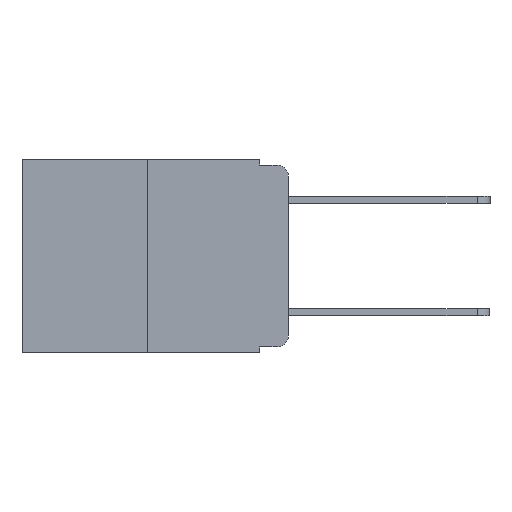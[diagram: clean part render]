
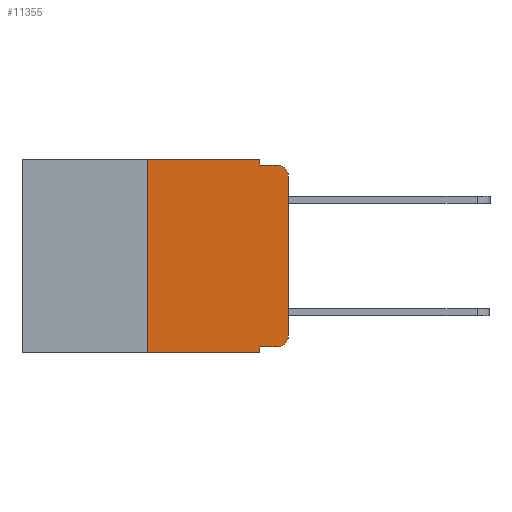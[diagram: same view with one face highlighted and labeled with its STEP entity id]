
A CAD part, left-side view. The second image highlights one B-rep face of the part: STEP entity #11355.
In plain terms, the highlighted planar face has unit normal (-1, 0, 0).
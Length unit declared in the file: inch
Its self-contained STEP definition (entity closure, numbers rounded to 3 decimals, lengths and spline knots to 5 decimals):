
#37 = ORIENTED_EDGE ( 'NONE', *, *, #12693, .T. ) ;
#157 = CARTESIAN_POINT ( 'NONE',  ( 0., 0.25, 0. ) ) ;
#374 = CARTESIAN_POINT ( 'NONE',  ( 0., 0.051, -0.01 ) ) ;
#707 = DIRECTION ( 'NONE',  ( 0., 0., -1. ) ) ;
#834 = CARTESIAN_POINT ( 'NONE',  ( 0., 0.02, -0.01 ) ) ;
#868 = EDGE_CURVE ( 'NONE', #13894, #13662, #4724, .T. ) ;
#949 = FACE_OUTER_BOUND ( 'NONE', #23629, .T. ) ;
#1075 = ORIENTED_EDGE ( 'NONE', *, *, #868, .F. ) ;
#1116 = VERTEX_POINT ( 'NONE', #12296 ) ;
#2257 = ORIENTED_EDGE ( 'NONE', *, *, #14462, .F. ) ;
#2414 = DIRECTION ( 'NONE',  ( 0., -1., 0. ) ) ;
#3928 = VERTEX_POINT ( 'NONE', #18220 ) ;
#4373 = LINE ( 'NONE', #13932, #23653 ) ;
#4468 = VECTOR ( 'NONE', #23866, 39.37008 ) ;
#4724 = LINE ( 'NONE', #21136, #17749 ) ;
#4776 = DIRECTION ( 'NONE',  ( -1., 0., 0. ) ) ;
#5752 = ORIENTED_EDGE ( 'NONE', *, *, #17588, .F. ) ;
#6073 = CIRCLE ( 'NONE', #23241, 0.02 ) ;
#6111 = VERTEX_POINT ( 'NONE', #834 ) ;
#6170 = ORIENTED_EDGE ( 'NONE', *, *, #16269, .T. ) ;
#6327 = DIRECTION ( 'NONE',  ( 1., 0., 0. ) ) ;
#6412 = CARTESIAN_POINT ( 'NONE',  ( 0., 0.473, 0. ) ) ;
#6756 = EDGE_CURVE ( 'NONE', #9820, #3928, #8186, .T. ) ;
#6792 = DIRECTION ( 'NONE',  ( 0., 0., 1. ) ) ;
#7317 = VERTEX_POINT ( 'NONE', #8262 ) ;
#7321 = VECTOR ( 'NONE', #14091, 39.37008 ) ;
#7469 = CIRCLE ( 'NONE', #14617, 0.02 ) ;
#7599 = VECTOR ( 'NONE', #707, 39.37008 ) ;
#7732 = DIRECTION ( 'NONE',  ( 0., 0., -1. ) ) ;
#8186 = LINE ( 'NONE', #16367, #7599 ) ;
#8262 = CARTESIAN_POINT ( 'NONE',  ( 0., 0.25, -0.343 ) ) ;
#8353 = PLANE ( 'NONE',  #20276 ) ;
#8526 = CARTESIAN_POINT ( 'NONE',  ( 0., 0.02, -0.03 ) ) ;
#8657 = EDGE_CURVE ( 'NONE', #7317, #3928, #4373, .T. ) ;
#8897 = ORIENTED_EDGE ( 'NONE', *, *, #8657, .T. ) ;
#9194 = DIRECTION ( 'NONE',  ( 0., -1., 0. ) ) ;
#9333 = EDGE_CURVE ( 'NONE', #7317, #13700, #9675, .T. ) ;
#9458 = VECTOR ( 'NONE', #2414, 39.37008 ) ;
#9675 = LINE ( 'NONE', #21959, #4468 ) ;
#9820 = VERTEX_POINT ( 'NONE', #17870 ) ;
#10146 = LINE ( 'NONE', #16385, #19770 ) ;
#10278 = DIRECTION ( 'NONE',  ( 0., 0., -1. ) ) ;
#10441 = DIRECTION ( 'NONE',  ( 0., 0., -1. ) ) ;
#11355 = ADVANCED_FACE ( 'NONE', ( #949 ), #8353, .F. ) ;
#11836 = CARTESIAN_POINT ( 'NONE',  ( 0., 0.051, -0.01 ) ) ;
#12060 = CARTESIAN_POINT ( 'NONE',  ( 0., 0.051, -0.333 ) ) ;
#12296 = CARTESIAN_POINT ( 'NONE',  ( 0., 0., -0.03 ) ) ;
#12315 = LINE ( 'NONE', #20678, #22527 ) ;
#12693 = EDGE_CURVE ( 'NONE', #12803, #1116, #10146, .T. ) ;
#12803 = VERTEX_POINT ( 'NONE', #12822 ) ;
#12822 = CARTESIAN_POINT ( 'NONE',  ( 0., 0., -0.313 ) ) ;
#13662 = VERTEX_POINT ( 'NONE', #11836 ) ;
#13700 = VERTEX_POINT ( 'NONE', #157 ) ;
#13894 = VERTEX_POINT ( 'NONE', #18333 ) ;
#13932 = CARTESIAN_POINT ( 'NONE',  ( 0., 0.473, -0.343 ) ) ;
#14091 = DIRECTION ( 'NONE',  ( 0., -1., 0. ) ) ;
#14462 = EDGE_CURVE ( 'NONE', #13662, #6111, #19677, .T. ) ;
#14525 = VERTEX_POINT ( 'NONE', #21883 ) ;
#14617 = AXIS2_PLACEMENT_3D ( 'NONE', #8526, #21932, #10441 ) ;
#16269 = EDGE_CURVE ( 'NONE', #9820, #14525, #18144, .T. ) ;
#16367 = CARTESIAN_POINT ( 'NONE',  ( 0., 0.051, 0. ) ) ;
#16382 = EDGE_CURVE ( 'NONE', #14525, #12803, #6073, .T. ) ;
#16385 = CARTESIAN_POINT ( 'NONE',  ( 0., 0., 0. ) ) ;
#16393 = CARTESIAN_POINT ( 'NONE',  ( 0., 0.02, -0.313 ) ) ;
#17588 = EDGE_CURVE ( 'NONE', #13700, #13894, #12315, .T. ) ;
#17749 = VECTOR ( 'NONE', #7732, 39.37008 ) ;
#17837 = DIRECTION ( 'NONE',  ( 0., -1., 0. ) ) ;
#17870 = CARTESIAN_POINT ( 'NONE',  ( 0., 0.051, -0.333 ) ) ;
#18144 = LINE ( 'NONE', #12060, #7321 ) ;
#18220 = CARTESIAN_POINT ( 'NONE',  ( 0., 0.051, -0.343 ) ) ;
#18308 = DIRECTION ( 'NONE',  ( 0., 0., -1. ) ) ;
#18333 = CARTESIAN_POINT ( 'NONE',  ( 0., 0.051, 0. ) ) ;
#18679 = ORIENTED_EDGE ( 'NONE', *, *, #19180, .T. ) ;
#18953 = ORIENTED_EDGE ( 'NONE', *, *, #9333, .F. ) ;
#19180 = EDGE_CURVE ( 'NONE', #1116, #6111, #7469, .T. ) ;
#19677 = LINE ( 'NONE', #374, #9458 ) ;
#19770 = VECTOR ( 'NONE', #6792, 39.37008 ) ;
#20019 = ORIENTED_EDGE ( 'NONE', *, *, #6756, .F. ) ;
#20276 = AXIS2_PLACEMENT_3D ( 'NONE', #6412, #6327, #10278 ) ;
#20678 = CARTESIAN_POINT ( 'NONE',  ( 0., 0.473, 0. ) ) ;
#21136 = CARTESIAN_POINT ( 'NONE',  ( 0., 0.051, 0. ) ) ;
#21883 = CARTESIAN_POINT ( 'NONE',  ( 0., 0.02, -0.333 ) ) ;
#21932 = DIRECTION ( 'NONE',  ( -1., 0., 0. ) ) ;
#21959 = CARTESIAN_POINT ( 'NONE',  ( 0., 0.25, 0. ) ) ;
#22527 = VECTOR ( 'NONE', #9194, 39.37008 ) ;
#23241 = AXIS2_PLACEMENT_3D ( 'NONE', #16393, #4776, #18308 ) ;
#23629 = EDGE_LOOP ( 'NONE', ( #37, #18679, #2257, #1075, #5752, #18953, #8897, #20019, #6170, #23851 ) ) ;
#23653 = VECTOR ( 'NONE', #17837, 39.37008 ) ;
#23851 = ORIENTED_EDGE ( 'NONE', *, *, #16382, .T. ) ;
#23866 = DIRECTION ( 'NONE',  ( 0., 0., 1. ) ) ;
